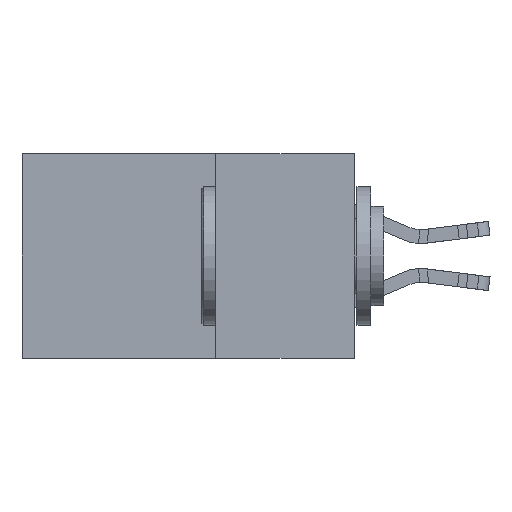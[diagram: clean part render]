
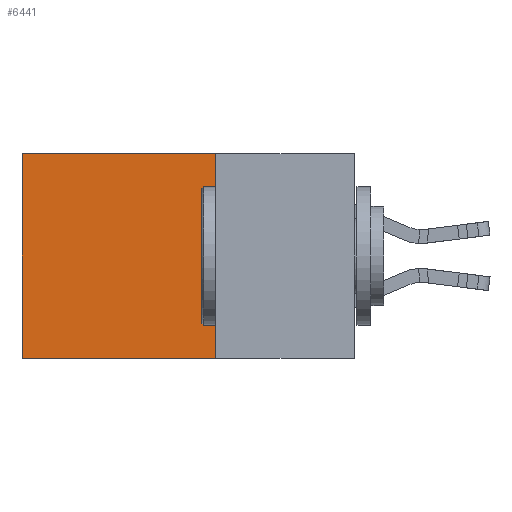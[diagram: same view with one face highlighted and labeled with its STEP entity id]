
A CAD part, left-side view. The second image highlights one B-rep face of the part: STEP entity #6441.
In plain terms, the highlighted planar face has unit normal (-1, 0, 0).
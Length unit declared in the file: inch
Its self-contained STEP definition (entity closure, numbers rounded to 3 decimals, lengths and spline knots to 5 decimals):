
#3923 = DIRECTION ( 'NONE',  ( 0., 1., 0. ) ) ;
#4646 = EDGE_CURVE ( 'NONE', #28957, #28758, #20762, .T. ) ;
#5179 = DIRECTION ( 'NONE',  ( 0., 0., -1. ) ) ;
#6441 = ADVANCED_FACE ( 'NONE', ( #10554 ), #16845, .F. ) ;
#6731 = CARTESIAN_POINT ( 'NONE',  ( 0.298, 0.25, -0.37 ) ) ;
#6910 = ORIENTED_EDGE ( 'NONE', *, *, #28844, .F. ) ;
#10407 = LINE ( 'NONE', #13354, #23919 ) ;
#10554 = FACE_OUTER_BOUND ( 'NONE', #14225, .T. ) ;
#10884 = VECTOR ( 'NONE', #3923, 39.37008 ) ;
#11524 = CARTESIAN_POINT ( 'NONE',  ( 0.298, 0.6, 0. ) ) ;
#13354 = CARTESIAN_POINT ( 'NONE',  ( 0.298, 0.25, -0.37 ) ) ;
#13677 = CARTESIAN_POINT ( 'NONE',  ( 0.298, 0.25, 0. ) ) ;
#14225 = EDGE_LOOP ( 'NONE', ( #16292, #6910, #14244, #17442 ) ) ;
#14244 = ORIENTED_EDGE ( 'NONE', *, *, #21283, .F. ) ;
#14362 = LINE ( 'NONE', #26078, #21832 ) ;
#14365 = DIRECTION ( 'NONE',  ( 0., 0., -1. ) ) ;
#14460 = VERTEX_POINT ( 'NONE', #21166 ) ;
#14854 = DIRECTION ( 'NONE',  ( 1., 0., 0. ) ) ;
#16292 = ORIENTED_EDGE ( 'NONE', *, *, #4646, .T. ) ;
#16845 = PLANE ( 'NONE',  #20140 ) ;
#17442 = ORIENTED_EDGE ( 'NONE', *, *, #27546, .T. ) ;
#18868 = DIRECTION ( 'NONE',  ( 0., 1., 0. ) ) ;
#19248 = CARTESIAN_POINT ( 'NONE',  ( 0.298, 0.25, 0. ) ) ;
#20140 = AXIS2_PLACEMENT_3D ( 'NONE', #19248, #14854, #5179 ) ;
#20762 = LINE ( 'NONE', #11524, #25990 ) ;
#21158 = DIRECTION ( 'NONE',  ( 0., 0., -1. ) ) ;
#21166 = CARTESIAN_POINT ( 'NONE',  ( 0.298, 0.25, 0. ) ) ;
#21283 = EDGE_CURVE ( 'NONE', #14460, #27853, #14362, .T. ) ;
#21832 = VECTOR ( 'NONE', #14365, 39.37008 ) ;
#22444 = CARTESIAN_POINT ( 'NONE',  ( 0.298, 0.6, -0.37 ) ) ;
#23893 = CARTESIAN_POINT ( 'NONE',  ( 0.298, 0.6, 0. ) ) ;
#23919 = VECTOR ( 'NONE', #18868, 39.37008 ) ;
#25990 = VECTOR ( 'NONE', #21158, 39.37008 ) ;
#26078 = CARTESIAN_POINT ( 'NONE',  ( 0.298, 0.25, 0. ) ) ;
#27546 = EDGE_CURVE ( 'NONE', #14460, #28957, #30362, .T. ) ;
#27853 = VERTEX_POINT ( 'NONE', #6731 ) ;
#28758 = VERTEX_POINT ( 'NONE', #22444 ) ;
#28844 = EDGE_CURVE ( 'NONE', #27853, #28758, #10407, .T. ) ;
#28957 = VERTEX_POINT ( 'NONE', #23893 ) ;
#30362 = LINE ( 'NONE', #13677, #10884 ) ;
